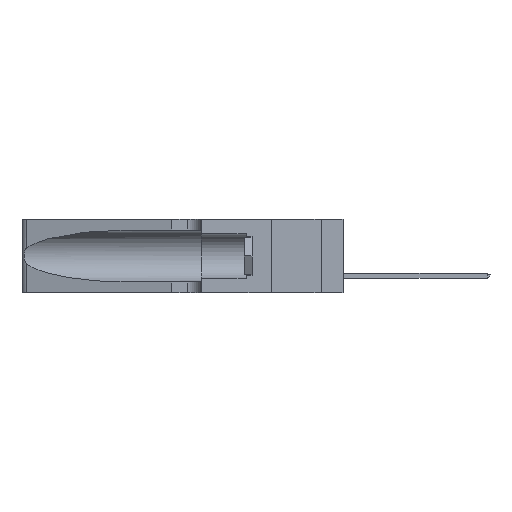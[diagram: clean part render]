
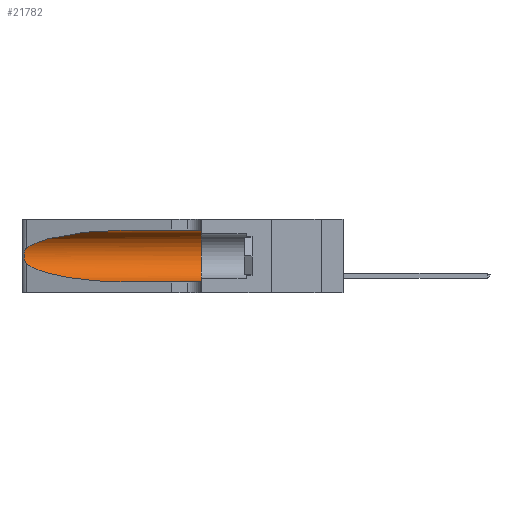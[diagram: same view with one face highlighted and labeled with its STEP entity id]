
A CAD part, left-side view. The second image highlights one B-rep face of the part: STEP entity #21782.
In plain terms, the highlighted cylindrical face has radius 3.308 mm (diameter 6.617 mm), a partial arc.
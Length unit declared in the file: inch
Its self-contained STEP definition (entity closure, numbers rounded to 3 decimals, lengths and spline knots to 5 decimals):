
#144 = VERTEX_POINT ( 'NONE', #25763 ) ;
#1578 = EDGE_CURVE ( 'NONE', #8626, #15148, #20596, .T. ) ;
#1868 = ORIENTED_EDGE ( 'NONE', *, *, #9156, .T. ) ;
#1940 = CARTESIAN_POINT ( 'NONE',  ( 0.25856, 1.23593, 0.16098 ) ) ;
#2144 = DIRECTION ( 'NONE',  ( 0., -1., 0. ) ) ;
#2201 = VECTOR ( 'NONE', #4926, 39.37008 ) ;
#3700 =( BOUNDED_CURVE ( )  B_SPLINE_CURVE ( 3, ( #36147, #6740, #27448, #28109 ),
 .UNSPECIFIED., .F., .T. ) 
 B_SPLINE_CURVE_WITH_KNOTS ( ( 4, 4 ),
 ( 3.44316, 4.71239 ),
 .UNSPECIFIED. ) 
 CURVE ( )  GEOMETRIC_REPRESENTATION_ITEM ( )  RATIONAL_B_SPLINE_CURVE ( ( 1., 0.87, 0.87, 1. ) ) 
 REPRESENTATION_ITEM ( '' )  );
#4170 = EDGE_CURVE ( 'NONE', #15148, #12280, #30870, .T. ) ;
#4560 = CARTESIAN_POINT ( 'NONE',  ( 0.25787, 1.23484, 0.2124 ) ) ;
#4926 = DIRECTION ( 'NONE',  ( 0., -1., 0. ) ) ;
#5115 = CARTESIAN_POINT ( 'NONE',  ( 0.26018, 1.23835, 0.19895 ) ) ;
#5527 = ORIENTED_EDGE ( 'NONE', *, *, #4170, .T. ) ;
#5631 = DIRECTION ( 'NONE',  ( 0., -1., 0. ) ) ;
#6256 = CYLINDRICAL_SURFACE ( 'NONE', #21014, 0.13025 ) ;
#6740 = CARTESIAN_POINT ( 'NONE',  ( 0.2373, 1.15595, 0.08982 ) ) ;
#7062 = CARTESIAN_POINT ( 'NONE',  ( 0.18966, 0.96281, 0.31525 ) ) ;
#7566 = ORIENTED_EDGE ( 'NONE', *, *, #16411, .T. ) ;
#8626 = VERTEX_POINT ( 'NONE', #32724 ) ;
#9156 = EDGE_CURVE ( 'NONE', #12280, #21157, #3700, .T. ) ;
#9516 = CARTESIAN_POINT ( 'NONE',  ( 0.1305, 0.72297, 0.05475 ) ) ;
#10052 = CARTESIAN_POINT ( 'NONE',  ( 0.25487, 1.22718, 0.22369 ) ) ;
#11207 = CARTESIAN_POINT ( 'NONE',  ( 0.26075, 1.23896, 0.19203 ) ) ;
#12280 = VERTEX_POINT ( 'NONE', #32923 ) ;
#13311 = CARTESIAN_POINT ( 'NONE',  ( 0.25487, 1.22718, 0.22369 ) ) ;
#13440 = CARTESIAN_POINT ( 'NONE',  ( 0.25639, 1.23184, 0.21858 ) ) ;
#13539 = CARTESIAN_POINT ( 'NONE',  ( 0.1305, 0.35, 0.05475 ) ) ;
#14025 = CARTESIAN_POINT ( 'NONE',  ( 0.1305, 1.61858, 0.185 ) ) ;
#14084 = CARTESIAN_POINT ( 'NONE',  ( 0.1305, 1.61858, 0.05475 ) ) ;
#14219 = CARTESIAN_POINT ( 'NONE',  ( 0.25555, 1.22993, 0.14849 ) ) ;
#15148 = VERTEX_POINT ( 'NONE', #21750 ) ;
#16411 = EDGE_CURVE ( 'NONE', #21157, #17019, #23728, .T. ) ;
#17019 = VERTEX_POINT ( 'NONE', #13539 ) ;
#17400 = AXIS2_PLACEMENT_3D ( 'NONE', #26510, #23605, #29645 ) ;
#19862 = CARTESIAN_POINT ( 'NONE',  ( 0.1305, 1.61858, 0.31525 ) ) ;
#20513 = CARTESIAN_POINT ( 'NONE',  ( 0.25487, 1.22718, 0.14631 ) ) ;
#20596 =( BOUNDED_CURVE ( )  B_SPLINE_CURVE ( 3, ( #33820, #7062, #28040, #10052 ),
 .UNSPECIFIED., .F., .F. ) 
 B_SPLINE_CURVE_WITH_KNOTS ( ( 4, 4 ),
 ( 1.5708, 2.84003 ),
 .UNSPECIFIED. ) 
 CURVE ( )  GEOMETRIC_REPRESENTATION_ITEM ( )  RATIONAL_B_SPLINE_CURVE ( ( 1., 0.87, 0.87, 1. ) ) 
 REPRESENTATION_ITEM ( '' )  );
#21014 = AXIS2_PLACEMENT_3D ( 'NONE', #14025, #5631, #32630 ) ;
#21157 = VERTEX_POINT ( 'NONE', #9516 ) ;
#21750 = CARTESIAN_POINT ( 'NONE',  ( 0.25487, 1.22718, 0.22369 ) ) ;
#21782 = ADVANCED_FACE ( 'NONE', ( #24507 ), #6256, .F. ) ;
#23135 = CIRCLE ( 'NONE', #17400, 0.13025 ) ;
#23605 = DIRECTION ( 'NONE',  ( 0., 1., 0. ) ) ;
#23728 = LINE ( 'NONE', #14084, #25607 ) ;
#24507 = FACE_OUTER_BOUND ( 'NONE', #29422, .T. ) ;
#25515 = CARTESIAN_POINT ( 'NONE',  ( 0.25854, 1.2359, 0.20912 ) ) ;
#25607 = VECTOR ( 'NONE', #2144, 39.37008 ) ;
#25763 = CARTESIAN_POINT ( 'NONE',  ( 0.1305, 0.35, 0.31525 ) ) ;
#25783 = CARTESIAN_POINT ( 'NONE',  ( 0.26017, 1.23833, 0.17102 ) ) ;
#26064 = CARTESIAN_POINT ( 'NONE',  ( 0.25789, 1.23486, 0.15765 ) ) ;
#26510 = CARTESIAN_POINT ( 'NONE',  ( 0.1305, 0.35, 0.185 ) ) ;
#27448 = CARTESIAN_POINT ( 'NONE',  ( 0.18966, 0.96281, 0.05475 ) ) ;
#27980 = CARTESIAN_POINT ( 'NONE',  ( 0.25555, 1.22994, 0.2215 ) ) ;
#28040 = CARTESIAN_POINT ( 'NONE',  ( 0.2373, 1.15595, 0.28018 ) ) ;
#28109 = CARTESIAN_POINT ( 'NONE',  ( 0.1305, 0.72297, 0.05475 ) ) ;
#28775 = ORIENTED_EDGE ( 'NONE', *, *, #30483, .F. ) ;
#29422 = EDGE_LOOP ( 'NONE', ( #30714, #5527, #1868, #7566, #28775, #30942 ) ) ;
#29645 = DIRECTION ( 'NONE',  ( 0., 0., 1. ) ) ;
#30483 = EDGE_CURVE ( 'NONE', #144, #17019, #23135, .T. ) ;
#30714 = ORIENTED_EDGE ( 'NONE', *, *, #1578, .T. ) ;
#30870 = B_SPLINE_CURVE_WITH_KNOTS ( 'NONE', 3,
 ( #13311, #27980, #13440, #4560, #25515, #5115, #11207, #37747, #25783, #1940, #26064, #31344, #14219, #20513 ),
 .UNSPECIFIED., .F., .F.,
 ( 4, 2, 2, 2, 2, 2, 4 ),
 ( 0., 0.00027, 0.00053, 0.00107, 0.0016, 0.00187, 0.00214 ),
 .UNSPECIFIED. ) ;
#30942 = ORIENTED_EDGE ( 'NONE', *, *, #38872, .F. ) ;
#31344 = CARTESIAN_POINT ( 'NONE',  ( 0.25639, 1.23186, 0.15144 ) ) ;
#32630 = DIRECTION ( 'NONE',  ( 0., 0., -1. ) ) ;
#32724 = CARTESIAN_POINT ( 'NONE',  ( 0.1305, 0.72297, 0.31525 ) ) ;
#32923 = CARTESIAN_POINT ( 'NONE',  ( 0.25487, 1.22718, 0.14631 ) ) ;
#33820 = CARTESIAN_POINT ( 'NONE',  ( 0.1305, 0.72297, 0.31525 ) ) ;
#36147 = CARTESIAN_POINT ( 'NONE',  ( 0.25487, 1.22718, 0.14631 ) ) ;
#36883 = LINE ( 'NONE', #19862, #2201 ) ;
#37747 = CARTESIAN_POINT ( 'NONE',  ( 0.26075, 1.23896, 0.178 ) ) ;
#38872 = EDGE_CURVE ( 'NONE', #8626, #144, #36883, .T. ) ;
